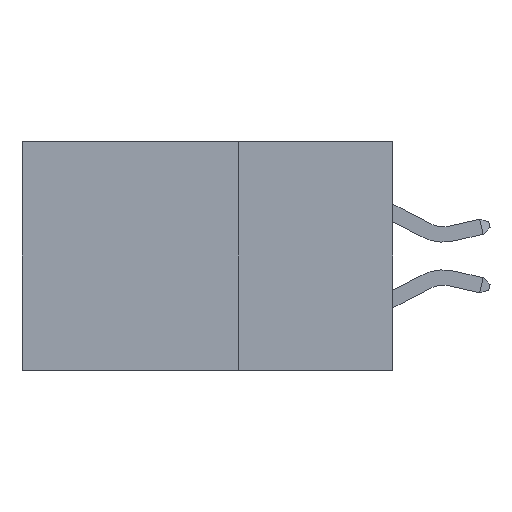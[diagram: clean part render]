
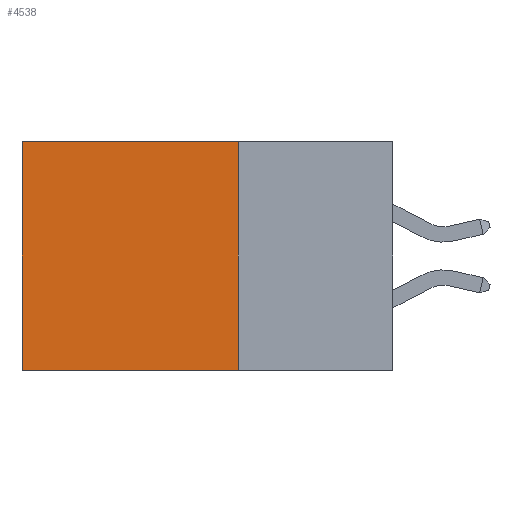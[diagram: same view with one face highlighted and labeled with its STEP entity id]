
A CAD part, left-side view. The second image highlights one B-rep face of the part: STEP entity #4538.
In plain terms, the highlighted planar face has unit normal (-1, 0, 0).
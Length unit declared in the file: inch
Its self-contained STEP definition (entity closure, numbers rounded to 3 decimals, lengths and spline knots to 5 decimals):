
#132 = EDGE_CURVE ( 'NONE', #14827, #9045, #3511, .T. ) ;
#1147 = LINE ( 'NONE', #13354, #14710 ) ;
#1822 = ORIENTED_EDGE ( 'NONE', *, *, #132, .T. ) ;
#3398 = LINE ( 'NONE', #6768, #10158 ) ;
#3511 = LINE ( 'NONE', #16373, #17145 ) ;
#4538 = ADVANCED_FACE ( 'NONE', ( #9305 ), #9419, .F. ) ;
#5140 = CARTESIAN_POINT ( 'NONE',  ( 0.2875, 0.6, 0. ) ) ;
#5498 = DIRECTION ( 'NONE',  ( 1., 0., 0. ) ) ;
#6148 = EDGE_CURVE ( 'NONE', #9045, #12238, #16730, .T. ) ;
#6296 = VECTOR ( 'NONE', #8203, 39.37008 ) ;
#6710 = EDGE_CURVE ( 'NONE', #17132, #12238, #1147, .T. ) ;
#6768 = CARTESIAN_POINT ( 'NONE',  ( 0.2875, 0.25, 0. ) ) ;
#8111 = DIRECTION ( 'NONE',  ( 0., 0., -1. ) ) ;
#8203 = DIRECTION ( 'NONE',  ( 0., 0., -1. ) ) ;
#9045 = VERTEX_POINT ( 'NONE', #5140 ) ;
#9305 = FACE_OUTER_BOUND ( 'NONE', #9699, .T. ) ;
#9419 = PLANE ( 'NONE',  #16040 ) ;
#9446 = DIRECTION ( 'NONE',  ( 0., 1., 0. ) ) ;
#9699 = EDGE_LOOP ( 'NONE', ( #14386, #13112, #12344, #1822 ) ) ;
#10158 = VECTOR ( 'NONE', #8111, 39.37008 ) ;
#12235 = EDGE_CURVE ( 'NONE', #14827, #17132, #3398, .T. ) ;
#12238 = VERTEX_POINT ( 'NONE', #14653 ) ;
#12344 = ORIENTED_EDGE ( 'NONE', *, *, #12235, .F. ) ;
#12615 = CARTESIAN_POINT ( 'NONE',  ( 0.2875, 0.25, 0. ) ) ;
#13112 = ORIENTED_EDGE ( 'NONE', *, *, #6710, .F. ) ;
#13354 = CARTESIAN_POINT ( 'NONE',  ( 0.2875, 0.25, -0.37 ) ) ;
#13384 = CARTESIAN_POINT ( 'NONE',  ( 0.2875, 0.25, 0. ) ) ;
#13829 = DIRECTION ( 'NONE',  ( 0., 1., 0. ) ) ;
#14386 = ORIENTED_EDGE ( 'NONE', *, *, #6148, .T. ) ;
#14653 = CARTESIAN_POINT ( 'NONE',  ( 0.2875, 0.6, -0.37 ) ) ;
#14685 = CARTESIAN_POINT ( 'NONE',  ( 0.2875, 0.6, 0. ) ) ;
#14696 = DIRECTION ( 'NONE',  ( 0., 0., -1. ) ) ;
#14710 = VECTOR ( 'NONE', #9446, 39.37008 ) ;
#14827 = VERTEX_POINT ( 'NONE', #12615 ) ;
#16040 = AXIS2_PLACEMENT_3D ( 'NONE', #13384, #5498, #14696 ) ;
#16373 = CARTESIAN_POINT ( 'NONE',  ( 0.2875, 0.25, 0. ) ) ;
#16730 = LINE ( 'NONE', #14685, #6296 ) ;
#17076 = CARTESIAN_POINT ( 'NONE',  ( 0.2875, 0.25, -0.37 ) ) ;
#17132 = VERTEX_POINT ( 'NONE', #17076 ) ;
#17145 = VECTOR ( 'NONE', #13829, 39.37008 ) ;
